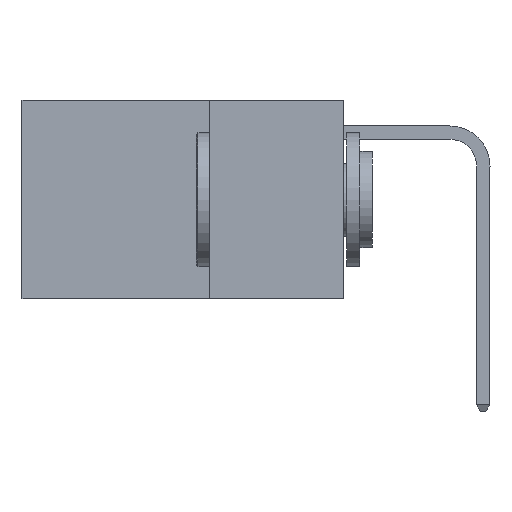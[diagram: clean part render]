
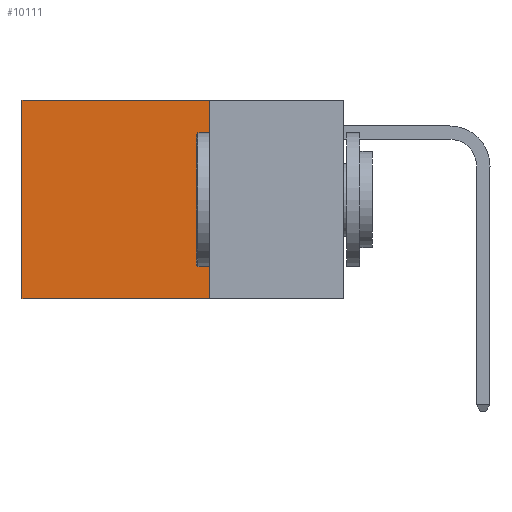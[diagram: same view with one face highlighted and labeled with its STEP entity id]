
A CAD part, left-side view. The second image highlights one B-rep face of the part: STEP entity #10111.
In plain terms, the highlighted planar face has unit normal (-1, 0, 0).
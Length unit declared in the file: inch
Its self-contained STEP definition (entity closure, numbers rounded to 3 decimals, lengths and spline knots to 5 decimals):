
#96 = VECTOR ( 'NONE', #1148, 39.37008 ) ;
#342 = ORIENTED_EDGE ( 'NONE', *, *, #11290, .T. ) ;
#392 = ORIENTED_EDGE ( 'NONE', *, *, #7257, .F. ) ;
#403 = ORIENTED_EDGE ( 'NONE', *, *, #8092, .F. ) ;
#445 = ORIENTED_EDGE ( 'NONE', *, *, #3715, .T. ) ;
#1148 = DIRECTION ( 'NONE',  ( 0., 0., -1. ) ) ;
#1466 = DIRECTION ( 'NONE',  ( 1., 0., 0. ) ) ;
#1656 = FACE_OUTER_BOUND ( 'NONE', #11423, .T. ) ;
#2055 = VERTEX_POINT ( 'NONE', #5083 ) ;
#2593 = CARTESIAN_POINT ( 'NONE',  ( 0.2625, 0.25, 0. ) ) ;
#2648 = DIRECTION ( 'NONE',  ( 0., 0., -1. ) ) ;
#3128 = VECTOR ( 'NONE', #9362, 39.37008 ) ;
#3280 = CARTESIAN_POINT ( 'NONE',  ( 0.2625, 0.25, -0.37 ) ) ;
#3715 = EDGE_CURVE ( 'NONE', #8780, #2055, #4003, .T. ) ;
#3755 = LINE ( 'NONE', #2593, #11437 ) ;
#4003 = LINE ( 'NONE', #4093, #6355 ) ;
#4010 = DIRECTION ( 'NONE',  ( 0., 1., 0. ) ) ;
#4093 = CARTESIAN_POINT ( 'NONE',  ( 0.2625, 0.25, 0. ) ) ;
#4953 = CARTESIAN_POINT ( 'NONE',  ( 0.2625, 0.25, -0.37 ) ) ;
#5083 = CARTESIAN_POINT ( 'NONE',  ( 0.2625, 0.6, 0. ) ) ;
#5124 = CARTESIAN_POINT ( 'NONE',  ( 0.2625, 0.6, -0.37 ) ) ;
#6157 = LINE ( 'NONE', #3280, #3128 ) ;
#6355 = VECTOR ( 'NONE', #4010, 39.37008 ) ;
#7257 = EDGE_CURVE ( 'NONE', #8231, #12265, #6157, .T. ) ;
#7691 = CARTESIAN_POINT ( 'NONE',  ( 0.2625, 0.25, 0. ) ) ;
#8092 = EDGE_CURVE ( 'NONE', #8780, #8231, #3755, .T. ) ;
#8231 = VERTEX_POINT ( 'NONE', #4953 ) ;
#8695 = DIRECTION ( 'NONE',  ( 0., 0., -1. ) ) ;
#8726 = LINE ( 'NONE', #11350, #96 ) ;
#8780 = VERTEX_POINT ( 'NONE', #12594 ) ;
#8912 = AXIS2_PLACEMENT_3D ( 'NONE', #7691, #1466, #8695 ) ;
#9362 = DIRECTION ( 'NONE',  ( 0., 1., 0. ) ) ;
#10111 = ADVANCED_FACE ( 'NONE', ( #1656 ), #11618, .F. ) ;
#11290 = EDGE_CURVE ( 'NONE', #2055, #12265, #8726, .T. ) ;
#11350 = CARTESIAN_POINT ( 'NONE',  ( 0.2625, 0.6, 0. ) ) ;
#11423 = EDGE_LOOP ( 'NONE', ( #342, #392, #403, #445 ) ) ;
#11437 = VECTOR ( 'NONE', #2648, 39.37008 ) ;
#11618 = PLANE ( 'NONE',  #8912 ) ;
#12265 = VERTEX_POINT ( 'NONE', #5124 ) ;
#12594 = CARTESIAN_POINT ( 'NONE',  ( 0.2625, 0.25, 0. ) ) ;
